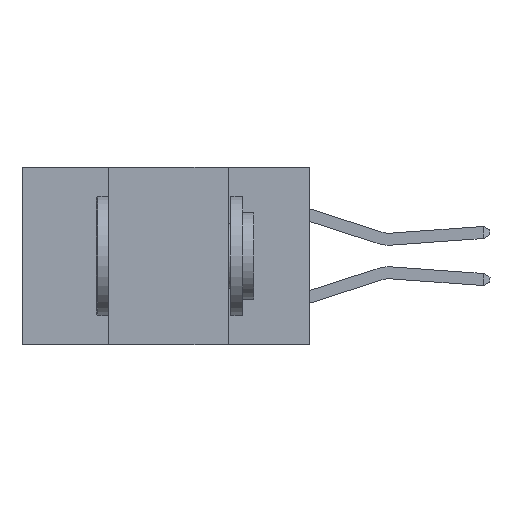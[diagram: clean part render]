
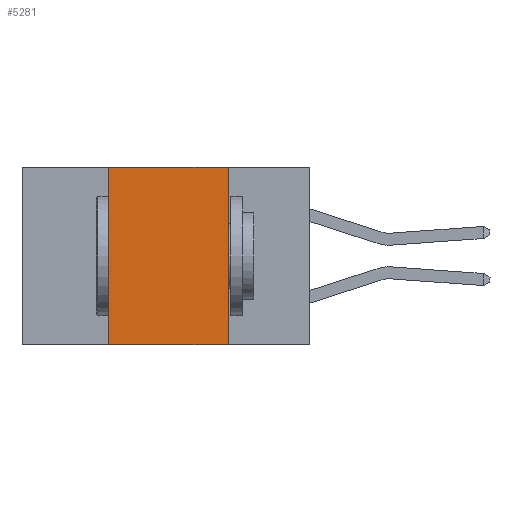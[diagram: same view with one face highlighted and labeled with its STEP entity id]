
A CAD part, left-side view. The second image highlights one B-rep face of the part: STEP entity #5281.
In plain terms, the highlighted planar face has unit normal (-1, 0, 0).
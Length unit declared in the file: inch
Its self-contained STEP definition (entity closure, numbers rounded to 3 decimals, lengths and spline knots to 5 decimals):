
#798 = VECTOR ( 'NONE', #14083, 39.37008 ) ;
#1431 = EDGE_CURVE ( 'NONE', #33734, #25833, #32092, .T. ) ;
#2158 = EDGE_CURVE ( 'NONE', #30110, #33734, #22138, .T. ) ;
#2346 = EDGE_CURVE ( 'NONE', #30110, #29254, #23779, .T. ) ;
#3011 = CARTESIAN_POINT ( 'NONE',  ( 0., 0.6, 0. ) ) ;
#4437 = CARTESIAN_POINT ( 'NONE',  ( 0., 0.6, -0.37 ) ) ;
#5281 = ADVANCED_FACE ( 'NONE', ( #12936 ), #10231, .F. ) ;
#6888 = DIRECTION ( 'NONE',  ( 0., -1., 0. ) ) ;
#8484 = ORIENTED_EDGE ( 'NONE', *, *, #2346, .T. ) ;
#8755 = CARTESIAN_POINT ( 'NONE',  ( 0., 0.42, 0. ) ) ;
#9027 = VECTOR ( 'NONE', #6888, 39.37008 ) ;
#10231 = PLANE ( 'NONE',  #33387 ) ;
#10905 = ORIENTED_EDGE ( 'NONE', *, *, #2158, .F. ) ;
#11131 = DIRECTION ( 'NONE',  ( 1., 0., 0. ) ) ;
#11208 = CARTESIAN_POINT ( 'NONE',  ( 0., 0.17, -0.37 ) ) ;
#12478 = CARTESIAN_POINT ( 'NONE',  ( 0., 0.42, -0.37 ) ) ;
#12936 = FACE_OUTER_BOUND ( 'NONE', #32625, .T. ) ;
#14083 = DIRECTION ( 'NONE',  ( 0., 0., -1. ) ) ;
#15209 = CARTESIAN_POINT ( 'NONE',  ( 0., 0.42, 0. ) ) ;
#19299 = ORIENTED_EDGE ( 'NONE', *, *, #33449, .F. ) ;
#22138 = LINE ( 'NONE', #8755, #22588 ) ;
#22265 = DIRECTION ( 'NONE',  ( 0., 0., 1. ) ) ;
#22588 = VECTOR ( 'NONE', #22265, 39.37008 ) ;
#23340 = CARTESIAN_POINT ( 'NONE',  ( 0., 0.17, 0. ) ) ;
#23779 = LINE ( 'NONE', #4437, #9027 ) ;
#24259 = LINE ( 'NONE', #29810, #798 ) ;
#25067 = VECTOR ( 'NONE', #26820, 39.37008 ) ;
#25379 = ORIENTED_EDGE ( 'NONE', *, *, #1431, .F. ) ;
#25833 = VERTEX_POINT ( 'NONE', #23340 ) ;
#26820 = DIRECTION ( 'NONE',  ( 0., -1., 0. ) ) ;
#26856 = CARTESIAN_POINT ( 'NONE',  ( 0., 0.6, 0. ) ) ;
#29254 = VERTEX_POINT ( 'NONE', #11208 ) ;
#29810 = CARTESIAN_POINT ( 'NONE',  ( 0., 0.17, 0. ) ) ;
#29850 = DIRECTION ( 'NONE',  ( 0., 0., -1. ) ) ;
#30110 = VERTEX_POINT ( 'NONE', #12478 ) ;
#32092 = LINE ( 'NONE', #3011, #25067 ) ;
#32625 = EDGE_LOOP ( 'NONE', ( #19299, #25379, #10905, #8484 ) ) ;
#33387 = AXIS2_PLACEMENT_3D ( 'NONE', #26856, #11131, #29850 ) ;
#33449 = EDGE_CURVE ( 'NONE', #25833, #29254, #24259, .T. ) ;
#33734 = VERTEX_POINT ( 'NONE', #15209 ) ;
